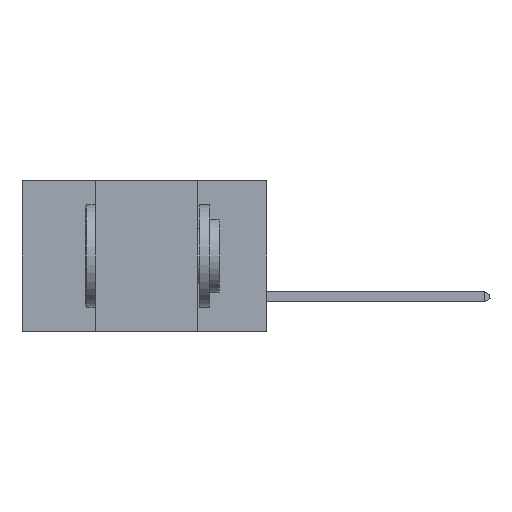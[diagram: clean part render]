
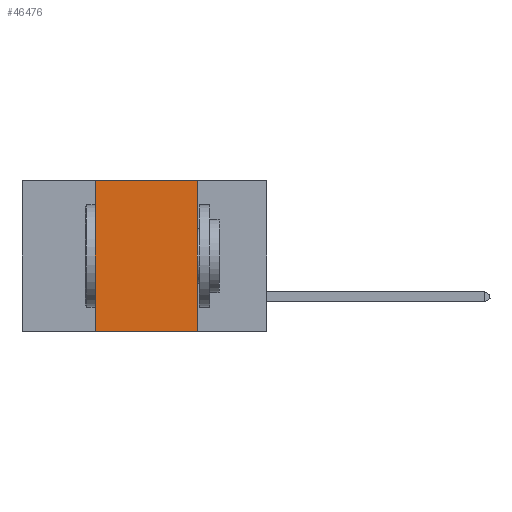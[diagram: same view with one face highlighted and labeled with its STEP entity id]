
A CAD part, left-side view. The second image highlights one B-rep face of the part: STEP entity #46476.
In plain terms, the highlighted planar face has unit normal (-1, 0, 0).
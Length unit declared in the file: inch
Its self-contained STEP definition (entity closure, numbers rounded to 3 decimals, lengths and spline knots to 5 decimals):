
#2064 = PLANE ( 'NONE',  #16018 ) ;
#4324 = EDGE_LOOP ( 'NONE', ( #20149, #8490, #16113, #41921 ) ) ;
#4370 = VERTEX_POINT ( 'NONE', #11504 ) ;
#4804 = CARTESIAN_POINT ( 'NONE',  ( 0., 0.6, 0. ) ) ;
#5521 = EDGE_CURVE ( 'NONE', #20780, #4370, #16610, .T. ) ;
#8490 = ORIENTED_EDGE ( 'NONE', *, *, #46550, .F. ) ;
#9526 = CARTESIAN_POINT ( 'NONE',  ( 0., 0.17, 0. ) ) ;
#9845 = FACE_OUTER_BOUND ( 'NONE', #4324, .T. ) ;
#11504 = CARTESIAN_POINT ( 'NONE',  ( 0., 0.42, 0. ) ) ;
#12489 = CARTESIAN_POINT ( 'NONE',  ( 0., 0.17, 0. ) ) ;
#13321 = DIRECTION ( 'NONE',  ( 0., -1., 0. ) ) ;
#13809 = VECTOR ( 'NONE', #13321, 39.37008 ) ;
#13894 = LINE ( 'NONE', #12489, #14453 ) ;
#14420 = LINE ( 'NONE', #47627, #13809 ) ;
#14453 = VECTOR ( 'NONE', #46967, 39.37008 ) ;
#15830 = DIRECTION ( 'NONE',  ( 0., 0., 1. ) ) ;
#16018 = AXIS2_PLACEMENT_3D ( 'NONE', #39735, #31638, #32346 ) ;
#16113 = ORIENTED_EDGE ( 'NONE', *, *, #5521, .F. ) ;
#16610 = LINE ( 'NONE', #30065, #33093 ) ;
#16647 = EDGE_CURVE ( 'NONE', #46895, #21902, #13894, .T. ) ;
#20149 = ORIENTED_EDGE ( 'NONE', *, *, #16647, .F. ) ;
#20780 = VERTEX_POINT ( 'NONE', #23299 ) ;
#21596 = LINE ( 'NONE', #4804, #26796 ) ;
#21902 = VERTEX_POINT ( 'NONE', #35681 ) ;
#23299 = CARTESIAN_POINT ( 'NONE',  ( 0., 0.42, -0.37 ) ) ;
#26796 = VECTOR ( 'NONE', #33841, 39.37008 ) ;
#30065 = CARTESIAN_POINT ( 'NONE',  ( 0., 0.42, 0. ) ) ;
#31638 = DIRECTION ( 'NONE',  ( 1., 0., 0. ) ) ;
#32346 = DIRECTION ( 'NONE',  ( 0., 0., -1. ) ) ;
#33093 = VECTOR ( 'NONE', #15830, 39.37008 ) ;
#33841 = DIRECTION ( 'NONE',  ( 0., -1., 0. ) ) ;
#35681 = CARTESIAN_POINT ( 'NONE',  ( 0., 0.17, -0.37 ) ) ;
#38732 = EDGE_CURVE ( 'NONE', #20780, #21902, #14420, .T. ) ;
#39735 = CARTESIAN_POINT ( 'NONE',  ( 0., 0.6, 0. ) ) ;
#41921 = ORIENTED_EDGE ( 'NONE', *, *, #38732, .T. ) ;
#46476 = ADVANCED_FACE ( 'NONE', ( #9845 ), #2064, .F. ) ;
#46550 = EDGE_CURVE ( 'NONE', #4370, #46895, #21596, .T. ) ;
#46895 = VERTEX_POINT ( 'NONE', #9526 ) ;
#46967 = DIRECTION ( 'NONE',  ( 0., 0., -1. ) ) ;
#47627 = CARTESIAN_POINT ( 'NONE',  ( 0., 0.6, -0.37 ) ) ;
